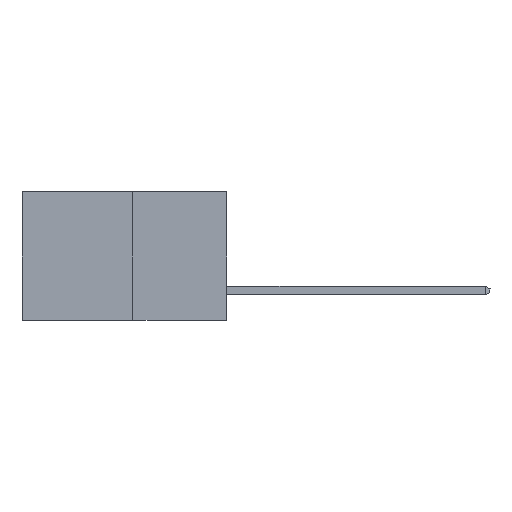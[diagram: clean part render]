
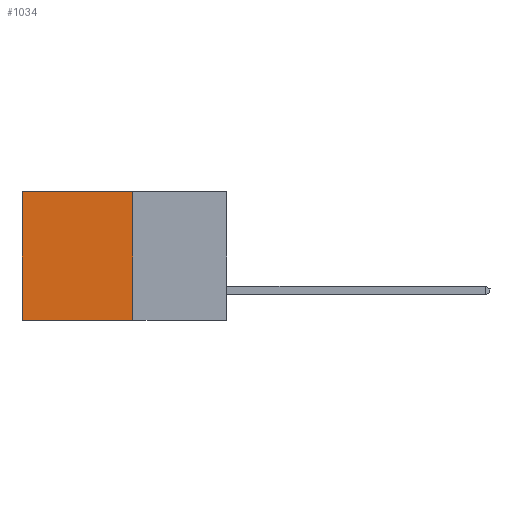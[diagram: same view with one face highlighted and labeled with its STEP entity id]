
A CAD part, left-side view. The second image highlights one B-rep face of the part: STEP entity #1034.
In plain terms, the highlighted planar face has unit normal (-1, 0, 0).
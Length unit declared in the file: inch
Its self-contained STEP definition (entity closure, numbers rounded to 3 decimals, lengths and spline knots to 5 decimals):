
#291 = LINE ( 'NONE', #2795, #10983 ) ;
#382 = PLANE ( 'NONE',  #7774 ) ;
#548 = DIRECTION ( 'NONE',  ( 1., 0., 0. ) ) ;
#710 = VERTEX_POINT ( 'NONE', #10802 ) ;
#1001 = VECTOR ( 'NONE', #6981, 39.37008 ) ;
#1034 = ADVANCED_FACE ( 'NONE', ( #9594 ), #382, .F. ) ;
#1298 = DIRECTION ( 'NONE',  ( 0., 0., -1. ) ) ;
#1448 = VERTEX_POINT ( 'NONE', #8008 ) ;
#1587 = DIRECTION ( 'NONE',  ( 0., 0., -1. ) ) ;
#1813 = CARTESIAN_POINT ( 'NONE',  ( 0.277, 0.27, -0.37 ) ) ;
#2412 = ORIENTED_EDGE ( 'NONE', *, *, #12635, .F. ) ;
#2795 = CARTESIAN_POINT ( 'NONE',  ( 0.277, 0.27, -0.37 ) ) ;
#2805 = ORIENTED_EDGE ( 'NONE', *, *, #11946, .F. ) ;
#2808 = CARTESIAN_POINT ( 'NONE',  ( 0.277, 0.27, 0. ) ) ;
#2810 = ORIENTED_EDGE ( 'NONE', *, *, #6650, .T. ) ;
#2864 = LINE ( 'NONE', #12985, #1001 ) ;
#3652 = VECTOR ( 'NONE', #1587, 39.37008 ) ;
#3786 = ORIENTED_EDGE ( 'NONE', *, *, #12658, .T. ) ;
#3855 = LINE ( 'NONE', #2808, #6633 ) ;
#4095 = DIRECTION ( 'NONE',  ( 0., 1., 0. ) ) ;
#4720 = VERTEX_POINT ( 'NONE', #9564 ) ;
#6633 = VECTOR ( 'NONE', #4095, 39.37008 ) ;
#6650 = EDGE_CURVE ( 'NONE', #710, #4720, #3855, .T. ) ;
#6778 = CARTESIAN_POINT ( 'NONE',  ( 0.277, 0.27, -0.37 ) ) ;
#6981 = DIRECTION ( 'NONE',  ( 0., 0., -1. ) ) ;
#7774 = AXIS2_PLACEMENT_3D ( 'NONE', #12260, #548, #1298 ) ;
#8008 = CARTESIAN_POINT ( 'NONE',  ( 0.277, 0.59, -0.37 ) ) ;
#9564 = CARTESIAN_POINT ( 'NONE',  ( 0.277, 0.59, 0. ) ) ;
#9594 = FACE_OUTER_BOUND ( 'NONE', #10712, .T. ) ;
#9729 = LINE ( 'NONE', #6778, #3652 ) ;
#10712 = EDGE_LOOP ( 'NONE', ( #3786, #2412, #2805, #2810 ) ) ;
#10802 = CARTESIAN_POINT ( 'NONE',  ( 0.277, 0.27, 0. ) ) ;
#10939 = DIRECTION ( 'NONE',  ( 0., 1., 0. ) ) ;
#10983 = VECTOR ( 'NONE', #10939, 39.37008 ) ;
#11946 = EDGE_CURVE ( 'NONE', #710, #12685, #9729, .T. ) ;
#12260 = CARTESIAN_POINT ( 'NONE',  ( 0.277, 0.27, -0.37 ) ) ;
#12635 = EDGE_CURVE ( 'NONE', #12685, #1448, #291, .T. ) ;
#12658 = EDGE_CURVE ( 'NONE', #4720, #1448, #2864, .T. ) ;
#12685 = VERTEX_POINT ( 'NONE', #1813 ) ;
#12985 = CARTESIAN_POINT ( 'NONE',  ( 0.277, 0.59, -0.37 ) ) ;
